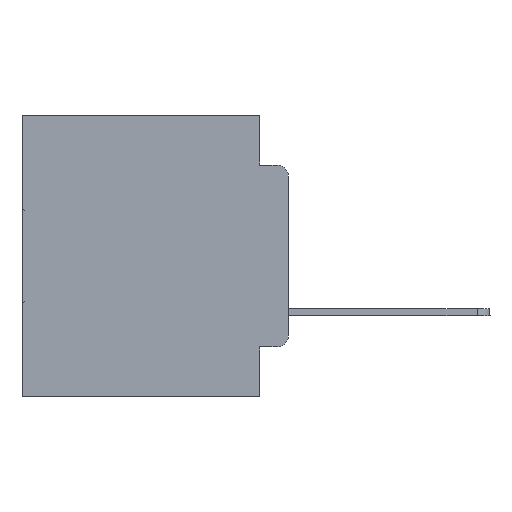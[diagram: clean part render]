
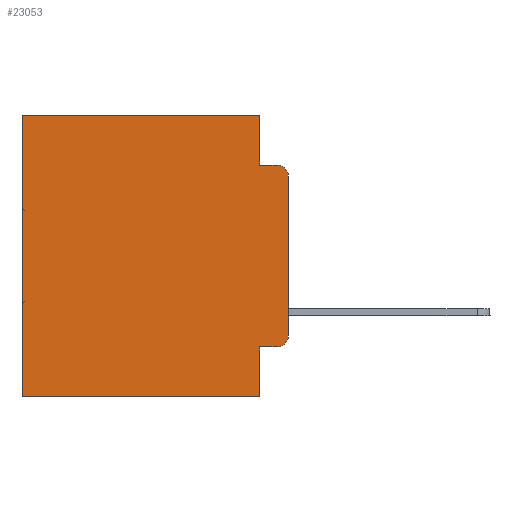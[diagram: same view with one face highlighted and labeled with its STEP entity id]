
A CAD part, left-side view. The second image highlights one B-rep face of the part: STEP entity #23053.
In plain terms, the highlighted planar face has unit normal (-1, 0, 0).
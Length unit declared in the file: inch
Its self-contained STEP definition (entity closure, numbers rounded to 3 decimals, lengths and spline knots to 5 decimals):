
#395 = DIRECTION ( 'NONE',  ( -1., 0., 0. ) ) ;
#426 = DIRECTION ( 'NONE',  ( 1., 0., 0. ) ) ;
#702 = EDGE_CURVE ( 'NONE', #3106, #14581, #16783, .T. ) ;
#725 = VECTOR ( 'NONE', #25303, 39.37008 ) ;
#2083 = VECTOR ( 'NONE', #7977, 39.37008 ) ;
#2178 = CARTESIAN_POINT ( 'NONE',  ( 0.298, 0., 0. ) ) ;
#2213 = CARTESIAN_POINT ( 'NONE',  ( 0.298, 0.051, -0.0885 ) ) ;
#2819 = DIRECTION ( 'NONE',  ( -1., 0., 0. ) ) ;
#3106 = VERTEX_POINT ( 'NONE', #13070 ) ;
#3287 = LINE ( 'NONE', #26912, #12681 ) ;
#3550 = CARTESIAN_POINT ( 'NONE',  ( 0.298, 0., -0.5 ) ) ;
#4943 = CARTESIAN_POINT ( 'NONE',  ( 0.298, 0.02, -0.4115 ) ) ;
#5178 = PLANE ( 'NONE',  #29776 ) ;
#5237 = AXIS2_PLACEMENT_3D ( 'NONE', #9946, #2819, #19854 ) ;
#5251 = LINE ( 'NONE', #3550, #725 ) ;
#5469 = CARTESIAN_POINT ( 'NONE',  ( 0.298, 0., -0.3915 ) ) ;
#5545 = VERTEX_POINT ( 'NONE', #27194 ) ;
#6250 = VECTOR ( 'NONE', #26394, 39.37008 ) ;
#6540 = EDGE_CURVE ( 'NONE', #29613, #9829, #8942, .T. ) ;
#6714 = EDGE_CURVE ( 'NONE', #17753, #14581, #21765, .T. ) ;
#7150 = VERTEX_POINT ( 'NONE', #19760 ) ;
#7480 = CARTESIAN_POINT ( 'NONE',  ( 0.298, 0., 0. ) ) ;
#7539 = DIRECTION ( 'NONE',  ( 0., -1., 0. ) ) ;
#7977 = DIRECTION ( 'NONE',  ( 0., 1., 0. ) ) ;
#8942 = LINE ( 'NONE', #19549, #9671 ) ;
#9480 = EDGE_CURVE ( 'NONE', #29613, #17780, #29524, .T. ) ;
#9671 = VECTOR ( 'NONE', #7539, 39.37008 ) ;
#9829 = VERTEX_POINT ( 'NONE', #4943 ) ;
#9865 = ORIENTED_EDGE ( 'NONE', *, *, #6540, .T. ) ;
#9946 = CARTESIAN_POINT ( 'NONE',  ( 0.298, 0.02, -0.3915 ) ) ;
#11361 = EDGE_CURVE ( 'NONE', #5545, #3106, #3287, .T. ) ;
#11679 = CARTESIAN_POINT ( 'NONE',  ( 0.298, 0.473, 0. ) ) ;
#12289 = CARTESIAN_POINT ( 'NONE',  ( 0.298, 0.051, -0.4115 ) ) ;
#12582 = DIRECTION ( 'NONE',  ( 0., 0., -1. ) ) ;
#12681 = VECTOR ( 'NONE', #12582, 39.37008 ) ;
#12878 = CARTESIAN_POINT ( 'NONE',  ( 0.298, 0.02, -0.0885 ) ) ;
#13070 = CARTESIAN_POINT ( 'NONE',  ( 0.298, 0.051, -0.0885 ) ) ;
#13515 = VECTOR ( 'NONE', #15694, 39.37008 ) ;
#14114 = DIRECTION ( 'NONE',  ( 0., 0., -1. ) ) ;
#14386 = ORIENTED_EDGE ( 'NONE', *, *, #6714, .T. ) ;
#14581 = VERTEX_POINT ( 'NONE', #12878 ) ;
#14652 = EDGE_CURVE ( 'NONE', #7150, #26810, #22706, .T. ) ;
#14976 = ORIENTED_EDGE ( 'NONE', *, *, #22804, .F. ) ;
#15694 = DIRECTION ( 'NONE',  ( 0., 0., -1. ) ) ;
#15877 = VECTOR ( 'NONE', #26771, 39.37008 ) ;
#16186 = CARTESIAN_POINT ( 'NONE',  ( 0.298, 0.473, -0.5 ) ) ;
#16783 = LINE ( 'NONE', #2213, #6250 ) ;
#16835 = VERTEX_POINT ( 'NONE', #5469 ) ;
#17151 = CARTESIAN_POINT ( 'NONE',  ( 0.298, 0.02, -0.1085 ) ) ;
#17237 = ORIENTED_EDGE ( 'NONE', *, *, #702, .F. ) ;
#17753 = VERTEX_POINT ( 'NONE', #22971 ) ;
#17780 = VERTEX_POINT ( 'NONE', #18173 ) ;
#18173 = CARTESIAN_POINT ( 'NONE',  ( 0.298, 0.051, -0.5 ) ) ;
#18491 = AXIS2_PLACEMENT_3D ( 'NONE', #17151, #395, #19572 ) ;
#18716 = EDGE_LOOP ( 'NONE', ( #18722, #14386, #17237, #21627, #21587, #21321, #14976, #19810, #9865, #19361 ) ) ;
#18722 = ORIENTED_EDGE ( 'NONE', *, *, #28247, .F. ) ;
#19361 = ORIENTED_EDGE ( 'NONE', *, *, #20546, .T. ) ;
#19549 = CARTESIAN_POINT ( 'NONE',  ( 0.298, 0.051, -0.4115 ) ) ;
#19572 = DIRECTION ( 'NONE',  ( 0., 0., -1. ) ) ;
#19760 = CARTESIAN_POINT ( 'NONE',  ( 0.298, 0.473, 0. ) ) ;
#19810 = ORIENTED_EDGE ( 'NONE', *, *, #9480, .F. ) ;
#19854 = DIRECTION ( 'NONE',  ( 0., 0., -1. ) ) ;
#19898 = LINE ( 'NONE', #27784, #13515 ) ;
#20546 = EDGE_CURVE ( 'NONE', #9829, #16835, #24675, .T. ) ;
#21321 = ORIENTED_EDGE ( 'NONE', *, *, #14652, .T. ) ;
#21587 = ORIENTED_EDGE ( 'NONE', *, *, #25135, .T. ) ;
#21627 = ORIENTED_EDGE ( 'NONE', *, *, #11361, .F. ) ;
#21765 = CIRCLE ( 'NONE', #18491, 0.02 ) ;
#21871 = CARTESIAN_POINT ( 'NONE',  ( 0.298, 0.051, 0. ) ) ;
#22706 = LINE ( 'NONE', #11679, #30281 ) ;
#22804 = EDGE_CURVE ( 'NONE', #17780, #26810, #5251, .T. ) ;
#22971 = CARTESIAN_POINT ( 'NONE',  ( 0.298, 0., -0.1085 ) ) ;
#23053 = ADVANCED_FACE ( 'NONE', ( #26774 ), #5178, .F. ) ;
#24310 = DIRECTION ( 'NONE',  ( 0., 0., -1. ) ) ;
#24675 = CIRCLE ( 'NONE', #5237, 0.02 ) ;
#25135 = EDGE_CURVE ( 'NONE', #5545, #7150, #31161, .T. ) ;
#25303 = DIRECTION ( 'NONE',  ( 0., 1., 0. ) ) ;
#26394 = DIRECTION ( 'NONE',  ( 0., -1., 0. ) ) ;
#26771 = DIRECTION ( 'NONE',  ( 0., 0., -1. ) ) ;
#26774 = FACE_OUTER_BOUND ( 'NONE', #18716, .T. ) ;
#26810 = VERTEX_POINT ( 'NONE', #16186 ) ;
#26912 = CARTESIAN_POINT ( 'NONE',  ( 0.298, 0.051, 0. ) ) ;
#27194 = CARTESIAN_POINT ( 'NONE',  ( 0.298, 0.051, 0. ) ) ;
#27784 = CARTESIAN_POINT ( 'NONE',  ( 0.298, 0., 0. ) ) ;
#28247 = EDGE_CURVE ( 'NONE', #17753, #16835, #19898, .T. ) ;
#29524 = LINE ( 'NONE', #21871, #15877 ) ;
#29613 = VERTEX_POINT ( 'NONE', #12289 ) ;
#29776 = AXIS2_PLACEMENT_3D ( 'NONE', #7480, #426, #24310 ) ;
#30281 = VECTOR ( 'NONE', #14114, 39.37008 ) ;
#31161 = LINE ( 'NONE', #2178, #2083 ) ;
